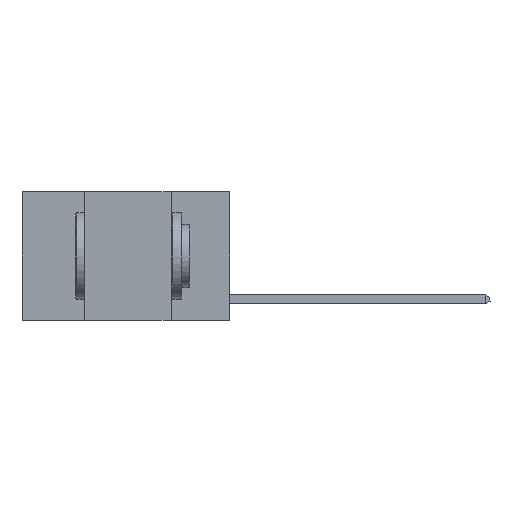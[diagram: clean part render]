
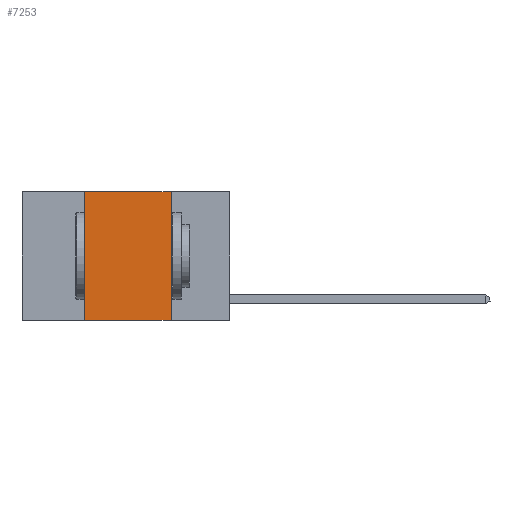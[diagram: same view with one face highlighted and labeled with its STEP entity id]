
A CAD part, left-side view. The second image highlights one B-rep face of the part: STEP entity #7253.
In plain terms, the highlighted planar face has unit normal (-1, 0, 0).
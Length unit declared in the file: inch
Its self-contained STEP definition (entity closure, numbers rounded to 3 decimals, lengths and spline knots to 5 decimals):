
#314 = ORIENTED_EDGE ( 'NONE', *, *, #14056, .T. ) ;
#1279 = CARTESIAN_POINT ( 'NONE',  ( 0., 0.42, 0. ) ) ;
#1740 = CARTESIAN_POINT ( 'NONE',  ( 0., 0.17, 0. ) ) ;
#1754 = CARTESIAN_POINT ( 'NONE',  ( 0., 0.6, 0. ) ) ;
#2375 = EDGE_CURVE ( 'NONE', #9334, #16284, #4255, .T. ) ;
#2396 = VECTOR ( 'NONE', #7966, 39.37008 ) ;
#2427 = VERTEX_POINT ( 'NONE', #14475 ) ;
#3247 = LINE ( 'NONE', #1754, #5075 ) ;
#3512 = CARTESIAN_POINT ( 'NONE',  ( 0., 0.17, 0. ) ) ;
#4255 = LINE ( 'NONE', #1279, #10742 ) ;
#4437 = DIRECTION ( 'NONE',  ( 1., 0., 0. ) ) ;
#5075 = VECTOR ( 'NONE', #6847, 39.37008 ) ;
#5878 = EDGE_CURVE ( 'NONE', #9180, #2427, #13900, .T. ) ;
#6198 = ORIENTED_EDGE ( 'NONE', *, *, #2375, .F. ) ;
#6847 = DIRECTION ( 'NONE',  ( 0., -1., 0. ) ) ;
#6921 = ORIENTED_EDGE ( 'NONE', *, *, #5878, .F. ) ;
#7253 = ADVANCED_FACE ( 'NONE', ( #8768 ), #13416, .F. ) ;
#7412 = EDGE_CURVE ( 'NONE', #16284, #9180, #3247, .T. ) ;
#7966 = DIRECTION ( 'NONE',  ( 0., 0., -1. ) ) ;
#8564 = ORIENTED_EDGE ( 'NONE', *, *, #7412, .F. ) ;
#8768 = FACE_OUTER_BOUND ( 'NONE', #13266, .T. ) ;
#8878 = DIRECTION ( 'NONE',  ( 0., 0., -1. ) ) ;
#9180 = VERTEX_POINT ( 'NONE', #3512 ) ;
#9334 = VERTEX_POINT ( 'NONE', #11268 ) ;
#9813 = CARTESIAN_POINT ( 'NONE',  ( 0., 0.42, 0. ) ) ;
#9998 = VECTOR ( 'NONE', #15386, 39.37008 ) ;
#10742 = VECTOR ( 'NONE', #13517, 39.37008 ) ;
#10812 = LINE ( 'NONE', #15104, #9998 ) ;
#11268 = CARTESIAN_POINT ( 'NONE',  ( 0., 0.42, -0.37 ) ) ;
#11907 = CARTESIAN_POINT ( 'NONE',  ( 0., 0.6, 0. ) ) ;
#12285 = AXIS2_PLACEMENT_3D ( 'NONE', #11907, #4437, #8878 ) ;
#13266 = EDGE_LOOP ( 'NONE', ( #6921, #8564, #6198, #314 ) ) ;
#13416 = PLANE ( 'NONE',  #12285 ) ;
#13517 = DIRECTION ( 'NONE',  ( 0., 0., 1. ) ) ;
#13900 = LINE ( 'NONE', #1740, #2396 ) ;
#14056 = EDGE_CURVE ( 'NONE', #9334, #2427, #10812, .T. ) ;
#14475 = CARTESIAN_POINT ( 'NONE',  ( 0., 0.17, -0.37 ) ) ;
#15104 = CARTESIAN_POINT ( 'NONE',  ( 0., 0.6, -0.37 ) ) ;
#15386 = DIRECTION ( 'NONE',  ( 0., -1., 0. ) ) ;
#16284 = VERTEX_POINT ( 'NONE', #9813 ) ;
